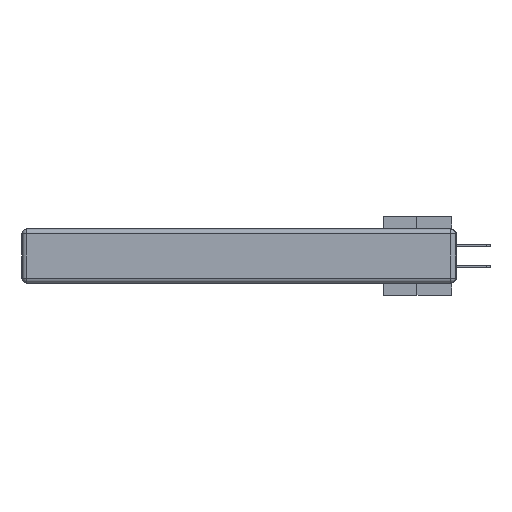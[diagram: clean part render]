
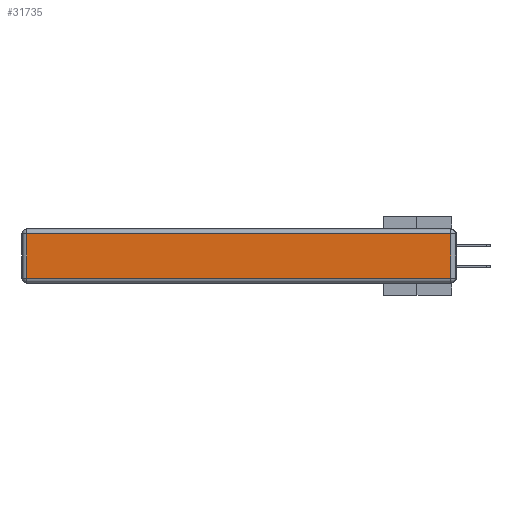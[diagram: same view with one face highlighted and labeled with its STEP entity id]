
A CAD part, left-side view. The second image highlights one B-rep face of the part: STEP entity #31735.
In plain terms, the highlighted planar face has unit normal (-1, 0, 0).
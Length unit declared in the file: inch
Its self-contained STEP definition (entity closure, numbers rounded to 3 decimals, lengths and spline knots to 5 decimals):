
#1500 = EDGE_LOOP ( 'NONE', ( #37362, #5166, #28217, #13788 ) ) ;
#2217 = CARTESIAN_POINT ( 'NONE',  ( 0., 0., -0.343 ) ) ;
#2524 = DIRECTION ( 'NONE',  ( -1., 0., 0. ) ) ;
#5166 = ORIENTED_EDGE ( 'NONE', *, *, #25805, .T. ) ;
#5535 = CARTESIAN_POINT ( 'NONE',  ( 0., 2.72, -0.313 ) ) ;
#6439 = DIRECTION ( 'NONE',  ( 0., 0., 1. ) ) ;
#7009 = VERTEX_POINT ( 'NONE', #33955 ) ;
#9089 = DIRECTION ( 'NONE',  ( 0., 0., 1. ) ) ;
#11420 = VERTEX_POINT ( 'NONE', #14667 ) ;
#12210 = EDGE_CURVE ( 'NONE', #29029, #11420, #22232, .T. ) ;
#12428 = DIRECTION ( 'NONE',  ( 0., 0., -1. ) ) ;
#12755 = VECTOR ( 'NONE', #14355, 39.37008 ) ;
#13466 = EDGE_CURVE ( 'NONE', #26847, #29029, #28772, .T. ) ;
#13788 = ORIENTED_EDGE ( 'NONE', *, *, #13466, .T. ) ;
#14355 = DIRECTION ( 'NONE',  ( 0., -1., 0. ) ) ;
#14667 = CARTESIAN_POINT ( 'NONE',  ( 0., 0.03, -0.313 ) ) ;
#16089 = CARTESIAN_POINT ( 'NONE',  ( 0., 2.75, -0.03 ) ) ;
#21927 = VECTOR ( 'NONE', #6439, 39.37008 ) ;
#22232 = LINE ( 'NONE', #35087, #12755 ) ;
#23336 = CARTESIAN_POINT ( 'NONE',  ( 0., 2.72, -0.343 ) ) ;
#24188 = LINE ( 'NONE', #45776, #21927 ) ;
#25037 = VECTOR ( 'NONE', #41021, 39.37008 ) ;
#25805 = EDGE_CURVE ( 'NONE', #11420, #7009, #24188, .T. ) ;
#26847 = VERTEX_POINT ( 'NONE', #27894 ) ;
#27894 = CARTESIAN_POINT ( 'NONE',  ( 0., 2.72, -0.03 ) ) ;
#28217 = ORIENTED_EDGE ( 'NONE', *, *, #42345, .T. ) ;
#28772 = LINE ( 'NONE', #23336, #37687 ) ;
#29029 = VERTEX_POINT ( 'NONE', #5535 ) ;
#31735 = ADVANCED_FACE ( 'NONE', ( #37269 ), #41206, .T. ) ;
#33955 = CARTESIAN_POINT ( 'NONE',  ( 0., 0.03, -0.03 ) ) ;
#35079 = LINE ( 'NONE', #16089, #25037 ) ;
#35087 = CARTESIAN_POINT ( 'NONE',  ( 0., 0., -0.313 ) ) ;
#37269 = FACE_OUTER_BOUND ( 'NONE', #1500, .T. ) ;
#37362 = ORIENTED_EDGE ( 'NONE', *, *, #12210, .T. ) ;
#37687 = VECTOR ( 'NONE', #12428, 39.37008 ) ;
#41021 = DIRECTION ( 'NONE',  ( 0., 1., 0. ) ) ;
#41206 = PLANE ( 'NONE',  #45797 ) ;
#42345 = EDGE_CURVE ( 'NONE', #7009, #26847, #35079, .T. ) ;
#45776 = CARTESIAN_POINT ( 'NONE',  ( 0., 0.03, -0.343 ) ) ;
#45797 = AXIS2_PLACEMENT_3D ( 'NONE', #2217, #2524, #9089 ) ;
